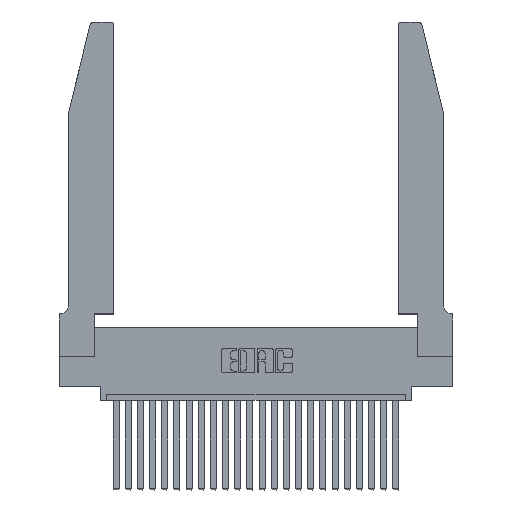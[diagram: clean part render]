
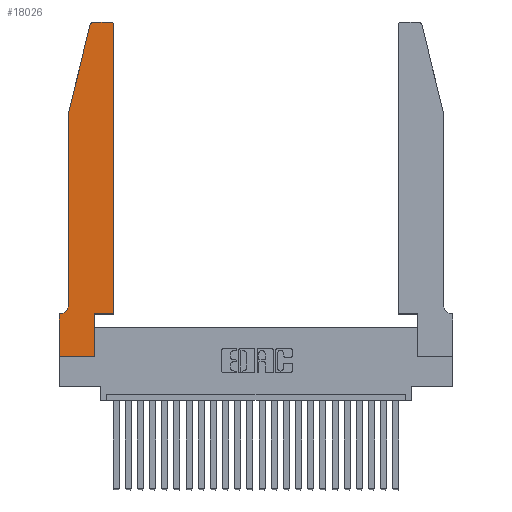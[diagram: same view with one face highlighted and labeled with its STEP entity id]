
A CAD part, top view. The second image highlights one B-rep face of the part: STEP entity #18026.
In plain terms, the highlighted planar face has unit normal (0, 0, 1).
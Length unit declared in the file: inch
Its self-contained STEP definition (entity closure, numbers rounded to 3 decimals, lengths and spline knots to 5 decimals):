
#120 = DIRECTION ( 'NONE',  ( -1., 0., 0. ) ) ;
#521 = EDGE_CURVE ( 'NONE', #16705, #23119, #16439, .T. ) ;
#721 = ORIENTED_EDGE ( 'NONE', *, *, #9512, .T. ) ;
#783 = CARTESIAN_POINT ( 'NONE',  ( 0.0055, 0.35, 0.37 ) ) ;
#939 = EDGE_CURVE ( 'NONE', #11323, #1753, #8512, .T. ) ;
#1020 = LINE ( 'NONE', #5918, #9796 ) ;
#1238 = LINE ( 'NONE', #17061, #11590 ) ;
#1327 = VERTEX_POINT ( 'NONE', #16863 ) ;
#1355 = DIRECTION ( 'NONE',  ( 0., 0., 1. ) ) ;
#1753 = VERTEX_POINT ( 'NONE', #15207 ) ;
#2398 = DIRECTION ( 'NONE',  ( -1., 0., 0. ) ) ;
#2495 = LINE ( 'NONE', #3554, #14656 ) ;
#2944 = AXIS2_PLACEMENT_3D ( 'NONE', #18082, #20027, #17904 ) ;
#3060 = DIRECTION ( 'NONE',  ( 1., 0., 0. ) ) ;
#3083 = LINE ( 'NONE', #5670, #23163 ) ;
#3131 = ORIENTED_EDGE ( 'NONE', *, *, #939, .T. ) ;
#3287 = CARTESIAN_POINT ( 'NONE',  ( 0.2865, 0.35, 0.37 ) ) ;
#3534 = DIRECTION ( 'NONE',  ( -0.239, -0.971, 0. ) ) ;
#3554 = CARTESIAN_POINT ( 'NONE',  ( 0.4505, 0.35, 0.37 ) ) ;
#3847 = CARTESIAN_POINT ( 'NONE',  ( 0.0755, 0.35, 0.37 ) ) ;
#4274 = VECTOR ( 'NONE', #3060, 39.37008 ) ;
#4708 = VERTEX_POINT ( 'NONE', #783 ) ;
#4867 = CARTESIAN_POINT ( 'NONE',  ( 0.0755, 2., 0.37 ) ) ;
#5670 = CARTESIAN_POINT ( 'NONE',  ( 0.2605, 2.75, 0.37 ) ) ;
#5800 = EDGE_CURVE ( 'NONE', #11979, #18634, #16953, .T. ) ;
#5918 = CARTESIAN_POINT ( 'NONE',  ( 0., 0., 0.37 ) ) ;
#6469 = VERTEX_POINT ( 'NONE', #10800 ) ;
#7342 = ORIENTED_EDGE ( 'NONE', *, *, #10524, .T. ) ;
#7381 = ORIENTED_EDGE ( 'NONE', *, *, #18141, .T. ) ;
#7424 = CARTESIAN_POINT ( 'NONE',  ( 0., 0., 0.37 ) ) ;
#7453 = DIRECTION ( 'NONE',  ( 1., 0., 0. ) ) ;
#7908 = CARTESIAN_POINT ( 'NONE',  ( 0.2865, 0.35, 0.37 ) ) ;
#8512 = CIRCLE ( 'NONE', #2944, 0.03 ) ;
#8776 = CARTESIAN_POINT ( 'NONE',  ( 0.2865, 0., 0.37 ) ) ;
#8922 = CARTESIAN_POINT ( 'NONE',  ( 0.4505, 0.35, 0.37 ) ) ;
#8923 = DIRECTION ( 'NONE',  ( 0., 0., -1. ) ) ;
#8944 = CARTESIAN_POINT ( 'NONE',  ( 0., 0., 0.37 ) ) ;
#9105 = AXIS2_PLACEMENT_3D ( 'NONE', #16565, #18612, #12670 ) ;
#9270 = ORIENTED_EDGE ( 'NONE', *, *, #10333, .T. ) ;
#9373 = CARTESIAN_POINT ( 'NONE',  ( 0.25487, 2.72718, 0.37 ) ) ;
#9482 = CIRCLE ( 'NONE', #17217, 0.03 ) ;
#9512 = EDGE_CURVE ( 'NONE', #6469, #4708, #19205, .T. ) ;
#9592 = VERTEX_POINT ( 'NONE', #16281 ) ;
#9796 = VECTOR ( 'NONE', #19515, 39.37008 ) ;
#10303 = PLANE ( 'NONE',  #9105 ) ;
#10333 = EDGE_CURVE ( 'NONE', #23119, #11323, #2495, .T. ) ;
#10388 = LINE ( 'NONE', #7908, #13706 ) ;
#10390 = AXIS2_PLACEMENT_3D ( 'NONE', #12746, #8923, #2398 ) ;
#10415 = EDGE_CURVE ( 'NONE', #1327, #13528, #9482, .T. ) ;
#10524 = EDGE_CURVE ( 'NONE', #1753, #1327, #3083, .T. ) ;
#10800 = CARTESIAN_POINT ( 'NONE',  ( 0.0755, 0.42, 0.37 ) ) ;
#11323 = VERTEX_POINT ( 'NONE', #16836 ) ;
#11374 = FACE_OUTER_BOUND ( 'NONE', #16692, .T. ) ;
#11590 = VECTOR ( 'NONE', #16891, 39.37008 ) ;
#11979 = VERTEX_POINT ( 'NONE', #7424 ) ;
#12670 = DIRECTION ( 'NONE',  ( 1., 0., 0. ) ) ;
#12746 = CARTESIAN_POINT ( 'NONE',  ( 0.0055, 0.42, 0.37 ) ) ;
#13268 = ORIENTED_EDGE ( 'NONE', *, *, #16096, .T. ) ;
#13528 = VERTEX_POINT ( 'NONE', #9373 ) ;
#13706 = VECTOR ( 'NONE', #21942, 39.37008 ) ;
#14656 = VECTOR ( 'NONE', #15383, 39.37008 ) ;
#14900 = ORIENTED_EDGE ( 'NONE', *, *, #5800, .T. ) ;
#14933 = CARTESIAN_POINT ( 'NONE',  ( 0.0755, 2., 0.37 ) ) ;
#15207 = CARTESIAN_POINT ( 'NONE',  ( 0.4205, 2.75, 0.37 ) ) ;
#15383 = DIRECTION ( 'NONE',  ( 0., 1., 0. ) ) ;
#15435 = EDGE_CURVE ( 'NONE', #4708, #9592, #21668, .T. ) ;
#15471 = VECTOR ( 'NONE', #21107, 39.37008 ) ;
#16096 = EDGE_CURVE ( 'NONE', #18634, #16705, #10388, .T. ) ;
#16167 = ORIENTED_EDGE ( 'NONE', *, *, #521, .T. ) ;
#16281 = CARTESIAN_POINT ( 'NONE',  ( 0., 0.35, 0.37 ) ) ;
#16366 = EDGE_CURVE ( 'NONE', #13528, #18020, #16725, .T. ) ;
#16439 = LINE ( 'NONE', #8922, #4274 ) ;
#16498 = VECTOR ( 'NONE', #120, 39.37008 ) ;
#16565 = CARTESIAN_POINT ( 'NONE',  ( 0., 0.35, 0.37 ) ) ;
#16692 = EDGE_LOOP ( 'NONE', ( #7342, #24674, #18966, #7381, #721, #22875, #18268, #14900, #13268, #16167, #9270, #3131 ) ) ;
#16705 = VERTEX_POINT ( 'NONE', #3287 ) ;
#16725 = LINE ( 'NONE', #14933, #17350 ) ;
#16836 = CARTESIAN_POINT ( 'NONE',  ( 0.4505, 2.72, 0.37 ) ) ;
#16863 = CARTESIAN_POINT ( 'NONE',  ( 0.284, 2.75, 0.37 ) ) ;
#16891 = DIRECTION ( 'NONE',  ( 0., -1., 0. ) ) ;
#16953 = LINE ( 'NONE', #8944, #15471 ) ;
#16975 = CARTESIAN_POINT ( 'NONE',  ( 0.4505, 0.35, 0.37 ) ) ;
#17061 = CARTESIAN_POINT ( 'NONE',  ( 0.0755, 2., 0.37 ) ) ;
#17217 = AXIS2_PLACEMENT_3D ( 'NONE', #22659, #1355, #7453 ) ;
#17350 = VECTOR ( 'NONE', #3534, 39.37008 ) ;
#17904 = DIRECTION ( 'NONE',  ( 1., 0., 0. ) ) ;
#18020 = VERTEX_POINT ( 'NONE', #4867 ) ;
#18026 = ADVANCED_FACE ( 'NONE', ( #11374 ), #10303, .T. ) ;
#18082 = CARTESIAN_POINT ( 'NONE',  ( 0.4205, 2.72, 0.37 ) ) ;
#18141 = EDGE_CURVE ( 'NONE', #18020, #6469, #1238, .T. ) ;
#18268 = ORIENTED_EDGE ( 'NONE', *, *, #23296, .T. ) ;
#18612 = DIRECTION ( 'NONE',  ( 0., 0., 1. ) ) ;
#18634 = VERTEX_POINT ( 'NONE', #8776 ) ;
#18966 = ORIENTED_EDGE ( 'NONE', *, *, #16366, .T. ) ;
#19205 = CIRCLE ( 'NONE', #10390, 0.07 ) ;
#19515 = DIRECTION ( 'NONE',  ( 0., -1., 0. ) ) ;
#20027 = DIRECTION ( 'NONE',  ( 0., 0., 1. ) ) ;
#21107 = DIRECTION ( 'NONE',  ( 1., 0., 0. ) ) ;
#21668 = LINE ( 'NONE', #3847, #16498 ) ;
#21942 = DIRECTION ( 'NONE',  ( 0., 1., 0. ) ) ;
#22659 = CARTESIAN_POINT ( 'NONE',  ( 0.284, 2.72, 0.37 ) ) ;
#22875 = ORIENTED_EDGE ( 'NONE', *, *, #15435, .T. ) ;
#23119 = VERTEX_POINT ( 'NONE', #16975 ) ;
#23163 = VECTOR ( 'NONE', #25183, 39.37008 ) ;
#23296 = EDGE_CURVE ( 'NONE', #9592, #11979, #1020, .T. ) ;
#24674 = ORIENTED_EDGE ( 'NONE', *, *, #10415, .T. ) ;
#25183 = DIRECTION ( 'NONE',  ( -1., 0., 0. ) ) ;
